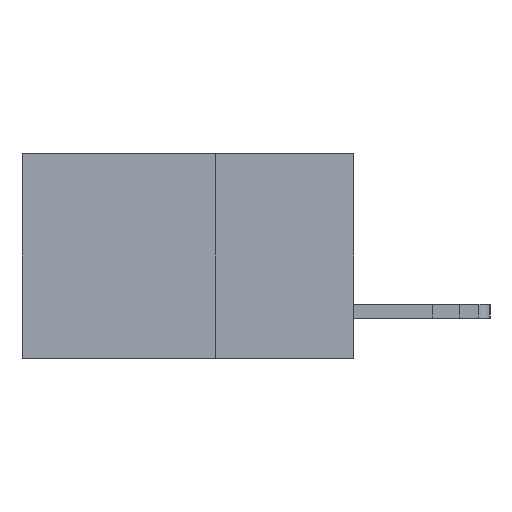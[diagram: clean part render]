
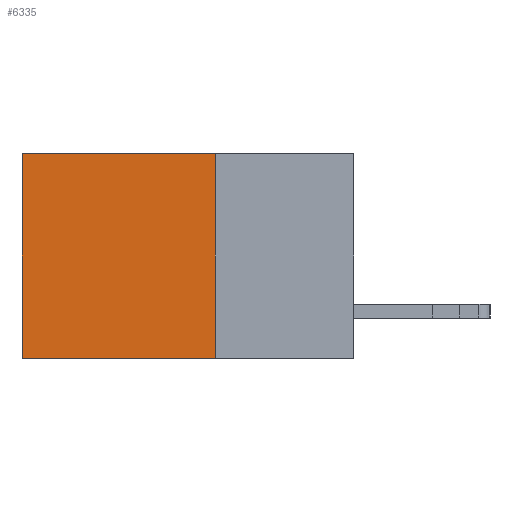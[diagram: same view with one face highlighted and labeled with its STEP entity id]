
A CAD part, left-side view. The second image highlights one B-rep face of the part: STEP entity #6335.
In plain terms, the highlighted planar face has unit normal (-1, 0, 0).
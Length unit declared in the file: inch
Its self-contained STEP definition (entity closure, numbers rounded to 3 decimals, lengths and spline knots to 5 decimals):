
#16 = CARTESIAN_POINT ( 'NONE',  ( 0.2875, 0.25, 0. ) ) ;
#178 = DIRECTION ( 'NONE',  ( 0., 0., -1. ) ) ;
#246 = EDGE_CURVE ( 'NONE', #9428, #6313, #9307, .T. ) ;
#597 = AXIS2_PLACEMENT_3D ( 'NONE', #1667, #14931, #178 ) ;
#1667 = CARTESIAN_POINT ( 'NONE',  ( 0.2875, 0.25, 0. ) ) ;
#2900 = CARTESIAN_POINT ( 'NONE',  ( 0.2875, 0.6, 0. ) ) ;
#3030 = CARTESIAN_POINT ( 'NONE',  ( 0.2875, 0.6, 0. ) ) ;
#3730 = VERTEX_POINT ( 'NONE', #12002 ) ;
#4090 = ORIENTED_EDGE ( 'NONE', *, *, #246, .T. ) ;
#4203 = LINE ( 'NONE', #12205, #16179 ) ;
#5022 = LINE ( 'NONE', #16, #11243 ) ;
#5353 = PLANE ( 'NONE',  #597 ) ;
#5441 = FACE_OUTER_BOUND ( 'NONE', #10361, .T. ) ;
#5604 = DIRECTION ( 'NONE',  ( 0., 1., 0. ) ) ;
#6292 = ORIENTED_EDGE ( 'NONE', *, *, #16051, .F. ) ;
#6313 = VERTEX_POINT ( 'NONE', #2900 ) ;
#6335 = ADVANCED_FACE ( 'NONE', ( #5441 ), #5353, .F. ) ;
#6495 = CARTESIAN_POINT ( 'NONE',  ( 0.2875, 0.25, 0. ) ) ;
#7325 = EDGE_CURVE ( 'NONE', #6313, #10575, #11376, .T. ) ;
#7365 = ORIENTED_EDGE ( 'NONE', *, *, #8079, .F. ) ;
#8079 = EDGE_CURVE ( 'NONE', #3730, #10575, #4203, .T. ) ;
#8597 = CARTESIAN_POINT ( 'NONE',  ( 0.2875, 0.25, 0. ) ) ;
#8659 = DIRECTION ( 'NONE',  ( 0., 0., -1. ) ) ;
#9307 = LINE ( 'NONE', #6495, #13376 ) ;
#9428 = VERTEX_POINT ( 'NONE', #8597 ) ;
#10361 = EDGE_LOOP ( 'NONE', ( #14710, #7365, #6292, #4090 ) ) ;
#10408 = VECTOR ( 'NONE', #8659, 39.37008 ) ;
#10575 = VERTEX_POINT ( 'NONE', #10889 ) ;
#10889 = CARTESIAN_POINT ( 'NONE',  ( 0.2875, 0.6, -0.37 ) ) ;
#11243 = VECTOR ( 'NONE', #15735, 39.37008 ) ;
#11376 = LINE ( 'NONE', #3030, #10408 ) ;
#12002 = CARTESIAN_POINT ( 'NONE',  ( 0.2875, 0.25, -0.37 ) ) ;
#12205 = CARTESIAN_POINT ( 'NONE',  ( 0.2875, 0.25, -0.37 ) ) ;
#13376 = VECTOR ( 'NONE', #15959, 39.37008 ) ;
#14710 = ORIENTED_EDGE ( 'NONE', *, *, #7325, .T. ) ;
#14931 = DIRECTION ( 'NONE',  ( 1., 0., 0. ) ) ;
#15735 = DIRECTION ( 'NONE',  ( 0., 0., -1. ) ) ;
#15959 = DIRECTION ( 'NONE',  ( 0., 1., 0. ) ) ;
#16051 = EDGE_CURVE ( 'NONE', #9428, #3730, #5022, .T. ) ;
#16179 = VECTOR ( 'NONE', #5604, 39.37008 ) ;
